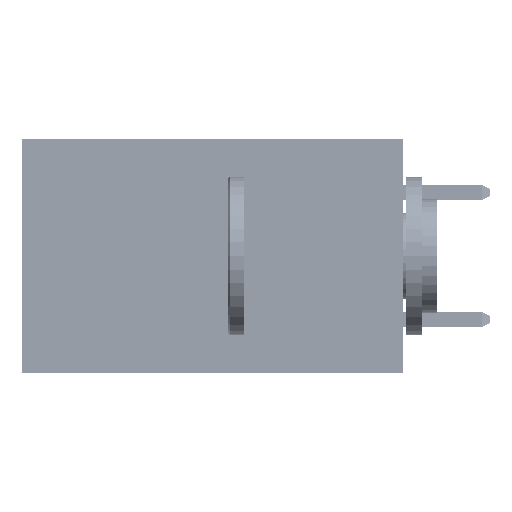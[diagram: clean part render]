
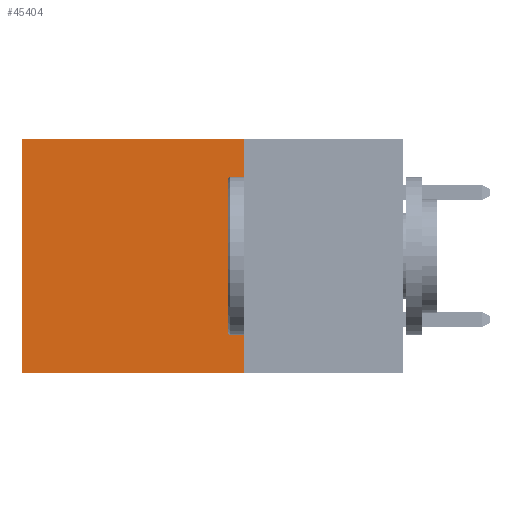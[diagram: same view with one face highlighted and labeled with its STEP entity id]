
A CAD part, left-side view. The second image highlights one B-rep face of the part: STEP entity #45404.
In plain terms, the highlighted planar face has unit normal (-1, 0, 0).
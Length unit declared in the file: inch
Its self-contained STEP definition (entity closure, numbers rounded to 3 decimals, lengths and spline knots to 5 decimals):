
#1112 = LINE ( 'NONE', #4568, #42564 ) ;
#4000 = VERTEX_POINT ( 'NONE', #42754 ) ;
#4568 = CARTESIAN_POINT ( 'NONE',  ( 0.2875, 0.25, -0.37 ) ) ;
#6728 = FACE_OUTER_BOUND ( 'NONE', #40525, .T. ) ;
#8339 = VECTOR ( 'NONE', #19004, 39.37008 ) ;
#8408 = EDGE_CURVE ( 'NONE', #25403, #4000, #28860, .T. ) ;
#8637 = DIRECTION ( 'NONE',  ( 0., 1., 0. ) ) ;
#9309 = ORIENTED_EDGE ( 'NONE', *, *, #19816, .F. ) ;
#10581 = ORIENTED_EDGE ( 'NONE', *, *, #33572, .F. ) ;
#11280 = ORIENTED_EDGE ( 'NONE', *, *, #8408, .T. ) ;
#15527 = DIRECTION ( 'NONE',  ( 1., 0., 0. ) ) ;
#15595 = DIRECTION ( 'NONE',  ( 0., 0., -1. ) ) ;
#16122 = CARTESIAN_POINT ( 'NONE',  ( 0.2875, 0.6, -0.37 ) ) ;
#17982 = CARTESIAN_POINT ( 'NONE',  ( 0.2875, 0.25, 0. ) ) ;
#18173 = VECTOR ( 'NONE', #22711, 39.37008 ) ;
#19004 = DIRECTION ( 'NONE',  ( 0., 0., -1. ) ) ;
#19816 = EDGE_CURVE ( 'NONE', #25403, #47031, #25899, .T. ) ;
#22711 = DIRECTION ( 'NONE',  ( 0., 1., 0. ) ) ;
#25017 = VERTEX_POINT ( 'NONE', #16122 ) ;
#25396 = CARTESIAN_POINT ( 'NONE',  ( 0.2875, 0.25, -0.37 ) ) ;
#25403 = VERTEX_POINT ( 'NONE', #17982 ) ;
#25899 = LINE ( 'NONE', #51532, #27178 ) ;
#27178 = VECTOR ( 'NONE', #15595, 39.37008 ) ;
#27494 = EDGE_CURVE ( 'NONE', #4000, #25017, #29658, .T. ) ;
#28860 = LINE ( 'NONE', #46470, #18173 ) ;
#29658 = LINE ( 'NONE', #46984, #8339 ) ;
#33572 = EDGE_CURVE ( 'NONE', #47031, #25017, #1112, .T. ) ;
#34703 = ORIENTED_EDGE ( 'NONE', *, *, #27494, .T. ) ;
#35543 = PLANE ( 'NONE',  #38094 ) ;
#38094 = AXIS2_PLACEMENT_3D ( 'NONE', #39554, #15527, #43518 ) ;
#39554 = CARTESIAN_POINT ( 'NONE',  ( 0.2875, 0.25, 0. ) ) ;
#40525 = EDGE_LOOP ( 'NONE', ( #34703, #10581, #9309, #11280 ) ) ;
#42564 = VECTOR ( 'NONE', #8637, 39.37008 ) ;
#42754 = CARTESIAN_POINT ( 'NONE',  ( 0.2875, 0.6, 0. ) ) ;
#43518 = DIRECTION ( 'NONE',  ( 0., 0., -1. ) ) ;
#45404 = ADVANCED_FACE ( 'NONE', ( #6728 ), #35543, .F. ) ;
#46470 = CARTESIAN_POINT ( 'NONE',  ( 0.2875, 0.25, 0. ) ) ;
#46984 = CARTESIAN_POINT ( 'NONE',  ( 0.2875, 0.6, 0. ) ) ;
#47031 = VERTEX_POINT ( 'NONE', #25396 ) ;
#51532 = CARTESIAN_POINT ( 'NONE',  ( 0.2875, 0.25, 0. ) ) ;
